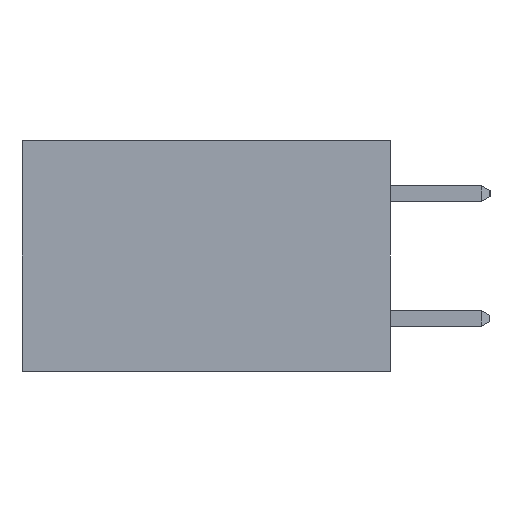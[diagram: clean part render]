
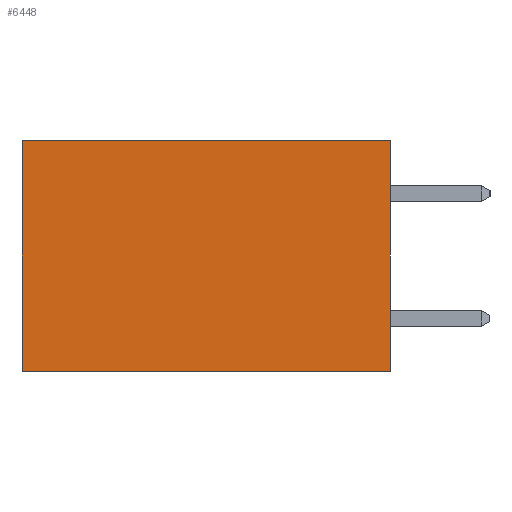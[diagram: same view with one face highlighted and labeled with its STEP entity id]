
A CAD part, left-side view. The second image highlights one B-rep face of the part: STEP entity #6448.
In plain terms, the highlighted planar face has unit normal (-1, 0, 0).
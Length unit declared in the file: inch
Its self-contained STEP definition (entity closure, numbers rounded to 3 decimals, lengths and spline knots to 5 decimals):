
#372 = VERTEX_POINT ( 'NONE', #566 ) ;
#566 = CARTESIAN_POINT ( 'NONE',  ( 0.277, 0., -0.37 ) ) ;
#637 = DIRECTION ( 'NONE',  ( 0., 1., 0. ) ) ;
#741 = CARTESIAN_POINT ( 'NONE',  ( 0.277, 0., 0. ) ) ;
#874 = VERTEX_POINT ( 'NONE', #13564 ) ;
#972 = LINE ( 'NONE', #10360, #4277 ) ;
#1487 = LINE ( 'NONE', #8355, #7032 ) ;
#1775 = EDGE_CURVE ( 'NONE', #2962, #14111, #12122, .T. ) ;
#1992 = VECTOR ( 'NONE', #10767, 39.37008 ) ;
#2799 = DIRECTION ( 'NONE',  ( 0., 1., 0. ) ) ;
#2962 = VERTEX_POINT ( 'NONE', #6054 ) ;
#3244 = VECTOR ( 'NONE', #2799, 39.37008 ) ;
#4222 = EDGE_LOOP ( 'NONE', ( #14265, #12637, #11191, #10434 ) ) ;
#4277 = VECTOR ( 'NONE', #10421, 39.37008 ) ;
#4413 = EDGE_CURVE ( 'NONE', #14111, #874, #10141, .T. ) ;
#4451 = EDGE_CURVE ( 'NONE', #2962, #372, #972, .T. ) ;
#5528 = DIRECTION ( 'NONE',  ( 0., 0., -1. ) ) ;
#5546 = DIRECTION ( 'NONE',  ( 1., 0., 0. ) ) ;
#5577 = CARTESIAN_POINT ( 'NONE',  ( 0.277, 0., -0.37 ) ) ;
#5800 = PLANE ( 'NONE',  #11142 ) ;
#6054 = CARTESIAN_POINT ( 'NONE',  ( 0.277, 0., 0. ) ) ;
#6448 = ADVANCED_FACE ( 'NONE', ( #12204 ), #5800, .F. ) ;
#7032 = VECTOR ( 'NONE', #637, 39.37008 ) ;
#8355 = CARTESIAN_POINT ( 'NONE',  ( 0.277, 0., -0.37 ) ) ;
#9381 = EDGE_CURVE ( 'NONE', #372, #874, #1487, .T. ) ;
#10141 = LINE ( 'NONE', #10869, #1992 ) ;
#10360 = CARTESIAN_POINT ( 'NONE',  ( 0.277, 0., -0.37 ) ) ;
#10421 = DIRECTION ( 'NONE',  ( 0., 0., -1. ) ) ;
#10434 = ORIENTED_EDGE ( 'NONE', *, *, #1775, .T. ) ;
#10767 = DIRECTION ( 'NONE',  ( 0., 0., -1. ) ) ;
#10869 = CARTESIAN_POINT ( 'NONE',  ( 0.277, 0.59, -0.37 ) ) ;
#11142 = AXIS2_PLACEMENT_3D ( 'NONE', #5577, #5546, #5528 ) ;
#11191 = ORIENTED_EDGE ( 'NONE', *, *, #4451, .F. ) ;
#11934 = CARTESIAN_POINT ( 'NONE',  ( 0.277, 0.59, 0. ) ) ;
#12122 = LINE ( 'NONE', #741, #3244 ) ;
#12204 = FACE_OUTER_BOUND ( 'NONE', #4222, .T. ) ;
#12637 = ORIENTED_EDGE ( 'NONE', *, *, #9381, .F. ) ;
#13564 = CARTESIAN_POINT ( 'NONE',  ( 0.277, 0.59, -0.37 ) ) ;
#14111 = VERTEX_POINT ( 'NONE', #11934 ) ;
#14265 = ORIENTED_EDGE ( 'NONE', *, *, #4413, .T. ) ;
